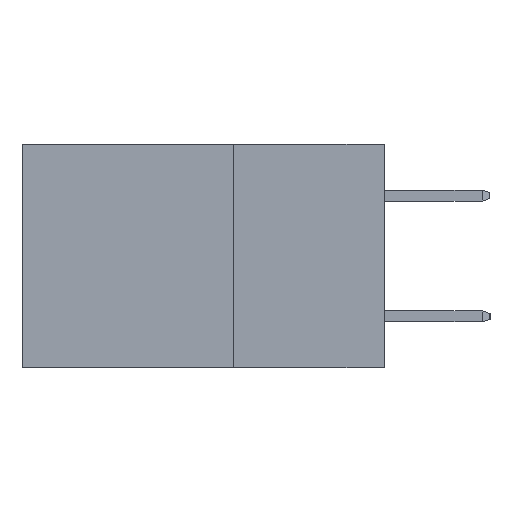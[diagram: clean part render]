
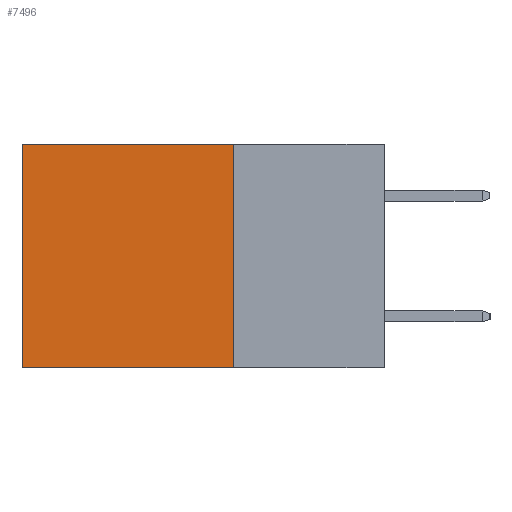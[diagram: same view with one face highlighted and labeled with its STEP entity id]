
A CAD part, left-side view. The second image highlights one B-rep face of the part: STEP entity #7496.
In plain terms, the highlighted planar face has unit normal (-1, 0, 0).
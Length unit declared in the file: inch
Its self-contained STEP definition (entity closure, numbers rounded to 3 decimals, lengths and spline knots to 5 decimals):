
#25 = EDGE_LOOP ( 'NONE', ( #1449, #12313, #4596, #12599 ) ) ;
#154 = CARTESIAN_POINT ( 'NONE',  ( 0.2615, 0.25, 0. ) ) ;
#807 = EDGE_CURVE ( 'NONE', #3519, #12915, #7154, .T. ) ;
#955 = DIRECTION ( 'NONE',  ( 0., 1., 0. ) ) ;
#1449 = ORIENTED_EDGE ( 'NONE', *, *, #8309, .T. ) ;
#2155 = VERTEX_POINT ( 'NONE', #9600 ) ;
#2681 = LINE ( 'NONE', #8289, #12752 ) ;
#3519 = VERTEX_POINT ( 'NONE', #7701 ) ;
#3687 = AXIS2_PLACEMENT_3D ( 'NONE', #3887, #3749, #3745 ) ;
#3745 = DIRECTION ( 'NONE',  ( 0., 0., -1. ) ) ;
#3748 = DIRECTION ( 'NONE',  ( 0., 0., -1. ) ) ;
#3749 = DIRECTION ( 'NONE',  ( 1., 0., 0. ) ) ;
#3763 = PLANE ( 'NONE',  #3687 ) ;
#3887 = CARTESIAN_POINT ( 'NONE',  ( 0.2615, 0.25, -0.37 ) ) ;
#4132 = CARTESIAN_POINT ( 'NONE',  ( 0.2615, 0.25, -0.37 ) ) ;
#4428 = EDGE_CURVE ( 'NONE', #12915, #9965, #10270, .T. ) ;
#4463 = FACE_OUTER_BOUND ( 'NONE', #25, .T. ) ;
#4596 = ORIENTED_EDGE ( 'NONE', *, *, #807, .F. ) ;
#4690 = LINE ( 'NONE', #154, #12391 ) ;
#7154 = LINE ( 'NONE', #11751, #12208 ) ;
#7496 = ADVANCED_FACE ( 'NONE', ( #4463 ), #3763, .F. ) ;
#7584 = VECTOR ( 'NONE', #955, 39.37008 ) ;
#7701 = CARTESIAN_POINT ( 'NONE',  ( 0.2615, 0.25, 0. ) ) ;
#8289 = CARTESIAN_POINT ( 'NONE',  ( 0.2615, 0.6, -0.37 ) ) ;
#8309 = EDGE_CURVE ( 'NONE', #2155, #9965, #2681, .T. ) ;
#8441 = DIRECTION ( 'NONE',  ( 0., 0., -1. ) ) ;
#8512 = DIRECTION ( 'NONE',  ( 0., 1., 0. ) ) ;
#8837 = CARTESIAN_POINT ( 'NONE',  ( 0.2615, 0.25, -0.37 ) ) ;
#9385 = CARTESIAN_POINT ( 'NONE',  ( 0.2615, 0.6, -0.37 ) ) ;
#9600 = CARTESIAN_POINT ( 'NONE',  ( 0.2615, 0.6, 0. ) ) ;
#9965 = VERTEX_POINT ( 'NONE', #9385 ) ;
#10270 = LINE ( 'NONE', #4132, #7584 ) ;
#11751 = CARTESIAN_POINT ( 'NONE',  ( 0.2615, 0.25, -0.37 ) ) ;
#12087 = EDGE_CURVE ( 'NONE', #3519, #2155, #4690, .T. ) ;
#12208 = VECTOR ( 'NONE', #3748, 39.37008 ) ;
#12313 = ORIENTED_EDGE ( 'NONE', *, *, #4428, .F. ) ;
#12391 = VECTOR ( 'NONE', #8512, 39.37008 ) ;
#12599 = ORIENTED_EDGE ( 'NONE', *, *, #12087, .T. ) ;
#12752 = VECTOR ( 'NONE', #8441, 39.37008 ) ;
#12915 = VERTEX_POINT ( 'NONE', #8837 ) ;
